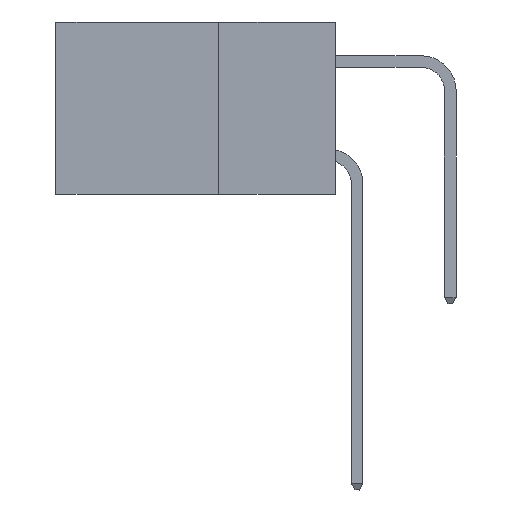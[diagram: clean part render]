
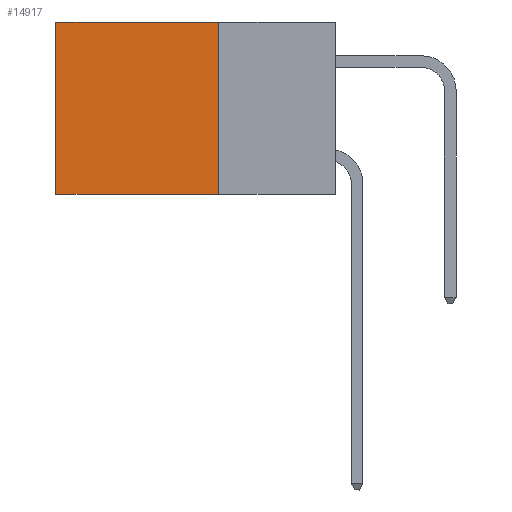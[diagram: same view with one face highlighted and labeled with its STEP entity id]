
A CAD part, left-side view. The second image highlights one B-rep face of the part: STEP entity #14917.
In plain terms, the highlighted planar face has unit normal (-1, 0, 0).
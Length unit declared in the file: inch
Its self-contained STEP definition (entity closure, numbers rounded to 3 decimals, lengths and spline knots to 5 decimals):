
#976 = CARTESIAN_POINT ( 'NONE',  ( 0.2875, 0.25, -0.37 ) ) ;
#1487 = ORIENTED_EDGE ( 'NONE', *, *, #7657, .T. ) ;
#1684 = VECTOR ( 'NONE', #19676, 39.37008 ) ;
#1943 = CARTESIAN_POINT ( 'NONE',  ( 0.2875, 0.25, 0. ) ) ;
#2797 = ORIENTED_EDGE ( 'NONE', *, *, #19283, .T. ) ;
#3565 = EDGE_CURVE ( 'NONE', #6957, #14538, #10713, .T. ) ;
#3910 = DIRECTION ( 'NONE',  ( 1., 0., 0. ) ) ;
#4050 = CARTESIAN_POINT ( 'NONE',  ( 0.2875, 0.6, -0.37 ) ) ;
#4502 = VECTOR ( 'NONE', #10784, 39.37008 ) ;
#6460 = VECTOR ( 'NONE', #12065, 39.37008 ) ;
#6957 = VERTEX_POINT ( 'NONE', #11203 ) ;
#7657 = EDGE_CURVE ( 'NONE', #6957, #19293, #9269, .T. ) ;
#8386 = CARTESIAN_POINT ( 'NONE',  ( 0.2875, 0.6, 0. ) ) ;
#8993 = CARTESIAN_POINT ( 'NONE',  ( 0.2875, 0.25, 0. ) ) ;
#9066 = DIRECTION ( 'NONE',  ( 0., 0., -1. ) ) ;
#9269 = LINE ( 'NONE', #12872, #4502 ) ;
#9317 = EDGE_LOOP ( 'NONE', ( #2797, #15247, #13795, #1487 ) ) ;
#10113 = LINE ( 'NONE', #17230, #21334 ) ;
#10574 = EDGE_CURVE ( 'NONE', #14538, #11222, #10113, .T. ) ;
#10713 = LINE ( 'NONE', #8993, #1684 ) ;
#10784 = DIRECTION ( 'NONE',  ( 0., 1., 0. ) ) ;
#11203 = CARTESIAN_POINT ( 'NONE',  ( 0.2875, 0.25, 0. ) ) ;
#11222 = VERTEX_POINT ( 'NONE', #4050 ) ;
#12065 = DIRECTION ( 'NONE',  ( 0., 0., -1. ) ) ;
#12762 = FACE_OUTER_BOUND ( 'NONE', #9317, .T. ) ;
#12872 = CARTESIAN_POINT ( 'NONE',  ( 0.2875, 0.25, 0. ) ) ;
#13564 = LINE ( 'NONE', #8386, #6460 ) ;
#13792 = DIRECTION ( 'NONE',  ( 0., 1., 0. ) ) ;
#13795 = ORIENTED_EDGE ( 'NONE', *, *, #3565, .F. ) ;
#14538 = VERTEX_POINT ( 'NONE', #976 ) ;
#14917 = ADVANCED_FACE ( 'NONE', ( #12762 ), #19635, .F. ) ;
#15247 = ORIENTED_EDGE ( 'NONE', *, *, #10574, .F. ) ;
#17223 = CARTESIAN_POINT ( 'NONE',  ( 0.2875, 0.6, 0. ) ) ;
#17230 = CARTESIAN_POINT ( 'NONE',  ( 0.2875, 0.25, -0.37 ) ) ;
#18471 = AXIS2_PLACEMENT_3D ( 'NONE', #1943, #3910, #9066 ) ;
#19283 = EDGE_CURVE ( 'NONE', #19293, #11222, #13564, .T. ) ;
#19293 = VERTEX_POINT ( 'NONE', #17223 ) ;
#19635 = PLANE ( 'NONE',  #18471 ) ;
#19676 = DIRECTION ( 'NONE',  ( 0., 0., -1. ) ) ;
#21334 = VECTOR ( 'NONE', #13792, 39.37008 ) ;
